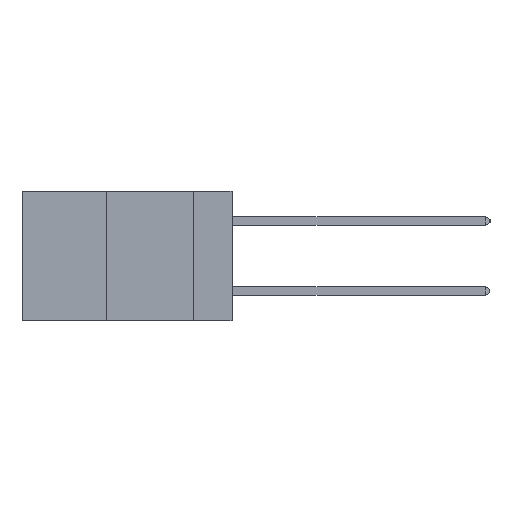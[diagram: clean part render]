
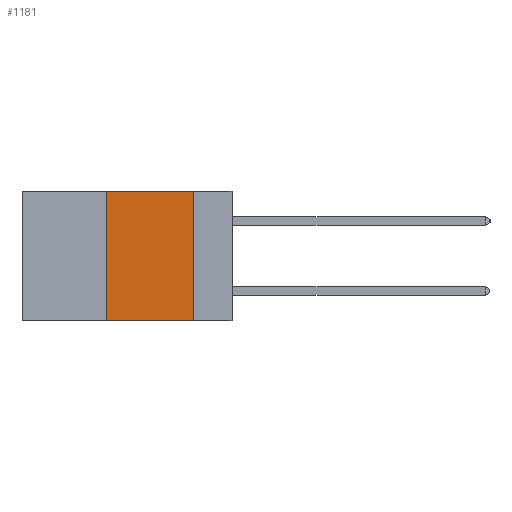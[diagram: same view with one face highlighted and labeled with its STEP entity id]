
A CAD part, left-side view. The second image highlights one B-rep face of the part: STEP entity #1181.
In plain terms, the highlighted planar face has unit normal (-1, 0, 0).
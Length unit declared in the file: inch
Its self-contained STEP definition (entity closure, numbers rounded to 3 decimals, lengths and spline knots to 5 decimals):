
#656 = VERTEX_POINT ( 'NONE', #17933 ) ;
#679 = ORIENTED_EDGE ( 'NONE', *, *, #10136, .F. ) ;
#1181 = ADVANCED_FACE ( 'NONE', ( #5567 ), #1256, .F. ) ;
#1199 = CARTESIAN_POINT ( 'NONE',  ( 0., 0.36, 0. ) ) ;
#1256 = PLANE ( 'NONE',  #10821 ) ;
#2104 = EDGE_CURVE ( 'NONE', #656, #13345, #17637, .T. ) ;
#2220 = CARTESIAN_POINT ( 'NONE',  ( 0., 0.6, 0. ) ) ;
#3064 = CARTESIAN_POINT ( 'NONE',  ( 0., 0.11, 0. ) ) ;
#3552 = VECTOR ( 'NONE', #6178, 39.37008 ) ;
#4449 = VECTOR ( 'NONE', #19579, 39.37008 ) ;
#5049 = LINE ( 'NONE', #17233, #18217 ) ;
#5567 = FACE_OUTER_BOUND ( 'NONE', #10404, .T. ) ;
#6178 = DIRECTION ( 'NONE',  ( 0., 0., -1. ) ) ;
#7099 = VERTEX_POINT ( 'NONE', #11646 ) ;
#8008 = DIRECTION ( 'NONE',  ( 0., 0., 1. ) ) ;
#8066 = LINE ( 'NONE', #20929, #3552 ) ;
#8725 = DIRECTION ( 'NONE',  ( 0., 0., -1. ) ) ;
#10136 = EDGE_CURVE ( 'NONE', #656, #7099, #14518, .T. ) ;
#10172 = VECTOR ( 'NONE', #8008, 39.37008 ) ;
#10404 = EDGE_LOOP ( 'NONE', ( #20258, #19082, #679, #18014 ) ) ;
#10821 = AXIS2_PLACEMENT_3D ( 'NONE', #2220, #19118, #8725 ) ;
#11110 = EDGE_CURVE ( 'NONE', #11237, #13345, #8066, .T. ) ;
#11237 = VERTEX_POINT ( 'NONE', #3064 ) ;
#11646 = CARTESIAN_POINT ( 'NONE',  ( 0., 0.36, 0. ) ) ;
#12384 = DIRECTION ( 'NONE',  ( 0., -1., 0. ) ) ;
#13345 = VERTEX_POINT ( 'NONE', #19126 ) ;
#13359 = CARTESIAN_POINT ( 'NONE',  ( 0., 0.6, -0.37 ) ) ;
#14518 = LINE ( 'NONE', #1199, #10172 ) ;
#17233 = CARTESIAN_POINT ( 'NONE',  ( 0., 0.6, 0. ) ) ;
#17637 = LINE ( 'NONE', #13359, #4449 ) ;
#17933 = CARTESIAN_POINT ( 'NONE',  ( 0., 0.36, -0.37 ) ) ;
#18014 = ORIENTED_EDGE ( 'NONE', *, *, #2104, .T. ) ;
#18217 = VECTOR ( 'NONE', #12384, 39.37008 ) ;
#19082 = ORIENTED_EDGE ( 'NONE', *, *, #19463, .F. ) ;
#19118 = DIRECTION ( 'NONE',  ( 1., 0., 0. ) ) ;
#19126 = CARTESIAN_POINT ( 'NONE',  ( 0., 0.11, -0.37 ) ) ;
#19463 = EDGE_CURVE ( 'NONE', #7099, #11237, #5049, .T. ) ;
#19579 = DIRECTION ( 'NONE',  ( 0., -1., 0. ) ) ;
#20258 = ORIENTED_EDGE ( 'NONE', *, *, #11110, .F. ) ;
#20929 = CARTESIAN_POINT ( 'NONE',  ( 0., 0.11, 0. ) ) ;
